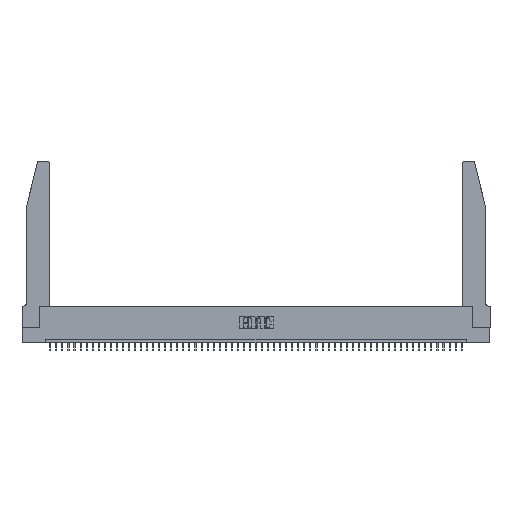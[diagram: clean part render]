
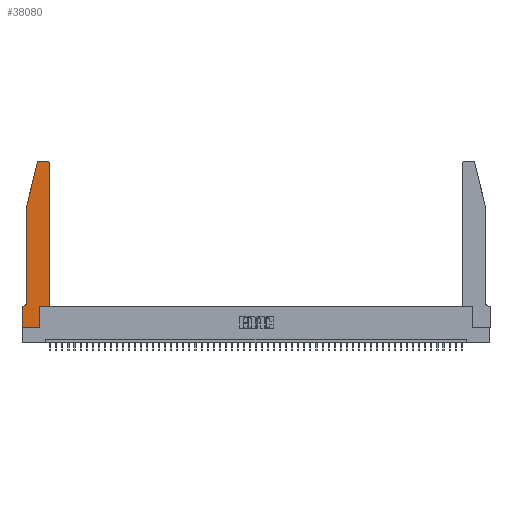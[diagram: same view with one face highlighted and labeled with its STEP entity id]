
A CAD part, top view. The second image highlights one B-rep face of the part: STEP entity #38080.
In plain terms, the highlighted planar face has unit normal (0, 0, 1).
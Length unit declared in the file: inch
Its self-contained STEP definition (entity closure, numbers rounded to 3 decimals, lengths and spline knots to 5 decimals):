
#101 = CARTESIAN_POINT ( 'NONE',  ( 0., 0.35, 0.37 ) ) ;
#297 = AXIS2_PLACEMENT_3D ( 'NONE', #17442, #9391, #16925 ) ;
#1051 = VECTOR ( 'NONE', #13928, 39.37008 ) ;
#1593 = FACE_OUTER_BOUND ( 'NONE', #44976, .T. ) ;
#1797 = DIRECTION ( 'NONE',  ( 0., 0., 1. ) ) ;
#1888 = ORIENTED_EDGE ( 'NONE', *, *, #42688, .T. ) ;
#2098 = VERTEX_POINT ( 'NONE', #37087 ) ;
#2195 = CARTESIAN_POINT ( 'NONE',  ( 0.2865, 0.35, 0.37 ) ) ;
#3124 = VECTOR ( 'NONE', #45842, 39.37008 ) ;
#3413 = CARTESIAN_POINT ( 'NONE',  ( 0.4205, 2.75, 0.37 ) ) ;
#4257 = DIRECTION ( 'NONE',  ( -1., 0., 0. ) ) ;
#4821 = VERTEX_POINT ( 'NONE', #101 ) ;
#5191 = AXIS2_PLACEMENT_3D ( 'NONE', #12846, #37009, #4257 ) ;
#5755 = DIRECTION ( 'NONE',  ( 1., 0., 0. ) ) ;
#6265 = LINE ( 'NONE', #38272, #8629 ) ;
#6729 = ORIENTED_EDGE ( 'NONE', *, *, #41213, .T. ) ;
#7076 = VECTOR ( 'NONE', #22209, 39.37008 ) ;
#8044 = CARTESIAN_POINT ( 'NONE',  ( 0.0755, 2., 0.37 ) ) ;
#8257 = VERTEX_POINT ( 'NONE', #45996 ) ;
#8411 = AXIS2_PLACEMENT_3D ( 'NONE', #30908, #42754, #38454 ) ;
#8629 = VECTOR ( 'NONE', #5755, 39.37008 ) ;
#9125 = LINE ( 'NONE', #38660, #1051 ) ;
#9391 = DIRECTION ( 'NONE',  ( 0., 0., 1. ) ) ;
#10380 = LINE ( 'NONE', #31053, #7076 ) ;
#10636 = EDGE_CURVE ( 'NONE', #17041, #4821, #46883, .T. ) ;
#12084 = ORIENTED_EDGE ( 'NONE', *, *, #36356, .T. ) ;
#12846 = CARTESIAN_POINT ( 'NONE',  ( 0.0055, 0.42, 0.37 ) ) ;
#13306 = LINE ( 'NONE', #42589, #24698 ) ;
#13928 = DIRECTION ( 'NONE',  ( 1., 0., 0. ) ) ;
#14442 = CARTESIAN_POINT ( 'NONE',  ( 0.4205, 2.72, 0.37 ) ) ;
#15161 = DIRECTION ( 'NONE',  ( -1., 0., 0. ) ) ;
#15778 = VERTEX_POINT ( 'NONE', #41695 ) ;
#16164 = CIRCLE ( 'NONE', #8411, 0.03 ) ;
#16446 = EDGE_CURVE ( 'NONE', #30262, #27482, #27611, .T. ) ;
#16925 = DIRECTION ( 'NONE',  ( 1., 0., 0. ) ) ;
#17041 = VERTEX_POINT ( 'NONE', #44998 ) ;
#17187 = PLANE ( 'NONE',  #297 ) ;
#17442 = CARTESIAN_POINT ( 'NONE',  ( 0., 0.35, 0.37 ) ) ;
#18177 = DIRECTION ( 'NONE',  ( 1., 0., 0. ) ) ;
#18289 = VERTEX_POINT ( 'NONE', #38436 ) ;
#18591 = DIRECTION ( 'NONE',  ( 0., 1., 0. ) ) ;
#19944 = VECTOR ( 'NONE', #20428, 39.37008 ) ;
#20428 = DIRECTION ( 'NONE',  ( -0.239, -0.971, 0. ) ) ;
#20927 = LINE ( 'NONE', #8044, #19944 ) ;
#22209 = DIRECTION ( 'NONE',  ( -1., 0., 0. ) ) ;
#22287 = EDGE_CURVE ( 'NONE', #4821, #46302, #13306, .T. ) ;
#23731 = VERTEX_POINT ( 'NONE', #3413 ) ;
#24698 = VECTOR ( 'NONE', #29427, 39.37008 ) ;
#25806 = EDGE_CURVE ( 'NONE', #23731, #18289, #10380, .T. ) ;
#27482 = VERTEX_POINT ( 'NONE', #41195 ) ;
#27611 = LINE ( 'NONE', #48572, #27805 ) ;
#27805 = VECTOR ( 'NONE', #48846, 39.37008 ) ;
#29427 = DIRECTION ( 'NONE',  ( 0., -1., 0. ) ) ;
#29712 = LINE ( 'NONE', #37787, #3124 ) ;
#29793 = VECTOR ( 'NONE', #18591, 39.37008 ) ;
#29977 = ORIENTED_EDGE ( 'NONE', *, *, #50697, .T. ) ;
#30262 = VERTEX_POINT ( 'NONE', #44028 ) ;
#30411 = LINE ( 'NONE', #2195, #29793 ) ;
#30908 = CARTESIAN_POINT ( 'NONE',  ( 0.284, 2.72, 0.37 ) ) ;
#31053 = CARTESIAN_POINT ( 'NONE',  ( 0.2605, 2.75, 0.37 ) ) ;
#32429 = ORIENTED_EDGE ( 'NONE', *, *, #49856, .T. ) ;
#33729 = CARTESIAN_POINT ( 'NONE',  ( 0.4505, 2.72, 0.37 ) ) ;
#36356 = EDGE_CURVE ( 'NONE', #8257, #2098, #9125, .T. ) ;
#37009 = DIRECTION ( 'NONE',  ( 0., 0., -1. ) ) ;
#37087 = CARTESIAN_POINT ( 'NONE',  ( 0.4505, 0.35, 0.37 ) ) ;
#37787 = CARTESIAN_POINT ( 'NONE',  ( 0.4505, 0.35, 0.37 ) ) ;
#37880 = ORIENTED_EDGE ( 'NONE', *, *, #22287, .T. ) ;
#38080 = ADVANCED_FACE ( 'NONE', ( #1593 ), #17187, .T. ) ;
#38272 = CARTESIAN_POINT ( 'NONE',  ( 0., 0., 0.37 ) ) ;
#38436 = CARTESIAN_POINT ( 'NONE',  ( 0.284, 2.75, 0.37 ) ) ;
#38454 = DIRECTION ( 'NONE',  ( 1., 0., 0. ) ) ;
#38660 = CARTESIAN_POINT ( 'NONE',  ( 0.4505, 0.35, 0.37 ) ) ;
#38867 = CARTESIAN_POINT ( 'NONE',  ( 0., 0., 0.37 ) ) ;
#40021 = AXIS2_PLACEMENT_3D ( 'NONE', #14442, #1797, #18177 ) ;
#40101 = VERTEX_POINT ( 'NONE', #45311 ) ;
#41195 = CARTESIAN_POINT ( 'NONE',  ( 0.0755, 0.42, 0.37 ) ) ;
#41213 = EDGE_CURVE ( 'NONE', #41567, #23731, #47780, .T. ) ;
#41567 = VERTEX_POINT ( 'NONE', #33729 ) ;
#41695 = CARTESIAN_POINT ( 'NONE',  ( 0.25487, 2.72718, 0.37 ) ) ;
#42046 = EDGE_CURVE ( 'NONE', #40101, #8257, #30411, .T. ) ;
#42589 = CARTESIAN_POINT ( 'NONE',  ( 0., 0., 0.37 ) ) ;
#42688 = EDGE_CURVE ( 'NONE', #2098, #41567, #29712, .T. ) ;
#42754 = DIRECTION ( 'NONE',  ( 0., 0., 1. ) ) ;
#44028 = CARTESIAN_POINT ( 'NONE',  ( 0.0755, 2., 0.37 ) ) ;
#44174 = ORIENTED_EDGE ( 'NONE', *, *, #25806, .T. ) ;
#44976 = EDGE_LOOP ( 'NONE', ( #44174, #49159, #29977, #49232, #51419, #47507, #37880, #32429, #48217, #12084, #1888, #6729 ) ) ;
#44998 = CARTESIAN_POINT ( 'NONE',  ( 0.0055, 0.35, 0.37 ) ) ;
#45051 = EDGE_CURVE ( 'NONE', #18289, #15778, #16164, .T. ) ;
#45311 = CARTESIAN_POINT ( 'NONE',  ( 0.2865, 0., 0.37 ) ) ;
#45842 = DIRECTION ( 'NONE',  ( 0., 1., 0. ) ) ;
#45996 = CARTESIAN_POINT ( 'NONE',  ( 0.2865, 0.35, 0.37 ) ) ;
#46302 = VERTEX_POINT ( 'NONE', #38867 ) ;
#46883 = LINE ( 'NONE', #47158, #47552 ) ;
#47158 = CARTESIAN_POINT ( 'NONE',  ( 0.0755, 0.35, 0.37 ) ) ;
#47507 = ORIENTED_EDGE ( 'NONE', *, *, #10636, .T. ) ;
#47552 = VECTOR ( 'NONE', #15161, 39.37008 ) ;
#47780 = CIRCLE ( 'NONE', #40021, 0.03 ) ;
#47912 = EDGE_CURVE ( 'NONE', #27482, #17041, #51524, .T. ) ;
#48217 = ORIENTED_EDGE ( 'NONE', *, *, #42046, .T. ) ;
#48572 = CARTESIAN_POINT ( 'NONE',  ( 0.0755, 2., 0.37 ) ) ;
#48846 = DIRECTION ( 'NONE',  ( 0., -1., 0. ) ) ;
#49159 = ORIENTED_EDGE ( 'NONE', *, *, #45051, .T. ) ;
#49232 = ORIENTED_EDGE ( 'NONE', *, *, #16446, .T. ) ;
#49856 = EDGE_CURVE ( 'NONE', #46302, #40101, #6265, .T. ) ;
#50697 = EDGE_CURVE ( 'NONE', #15778, #30262, #20927, .T. ) ;
#51419 = ORIENTED_EDGE ( 'NONE', *, *, #47912, .T. ) ;
#51524 = CIRCLE ( 'NONE', #5191, 0.07 ) ;
